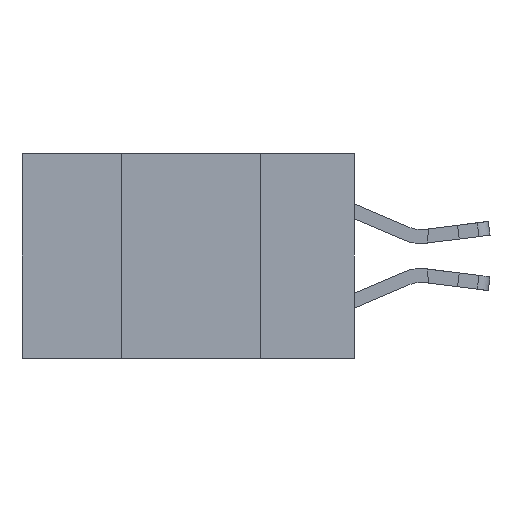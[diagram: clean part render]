
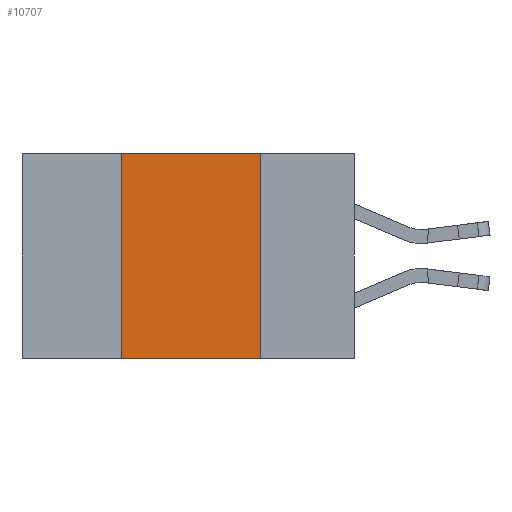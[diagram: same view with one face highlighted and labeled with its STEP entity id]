
A CAD part, left-side view. The second image highlights one B-rep face of the part: STEP entity #10707.
In plain terms, the highlighted planar face has unit normal (-1, 0, 0).
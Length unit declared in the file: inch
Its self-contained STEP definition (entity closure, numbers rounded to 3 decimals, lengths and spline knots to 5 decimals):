
#475 = VERTEX_POINT ( 'NONE', #1895 ) ;
#524 = CARTESIAN_POINT ( 'NONE',  ( 0., 0.42, -0.37 ) ) ;
#1473 = ORIENTED_EDGE ( 'NONE', *, *, #10453, .F. ) ;
#1657 = CARTESIAN_POINT ( 'NONE',  ( 0., 0.6, 0. ) ) ;
#1805 = FACE_OUTER_BOUND ( 'NONE', #2072, .T. ) ;
#1867 = ORIENTED_EDGE ( 'NONE', *, *, #7576, .F. ) ;
#1895 = CARTESIAN_POINT ( 'NONE',  ( 0., 0.17, 0. ) ) ;
#2072 = EDGE_LOOP ( 'NONE', ( #7737, #1867, #1473, #7550 ) ) ;
#2211 = LINE ( 'NONE', #5870, #7293 ) ;
#2310 = AXIS2_PLACEMENT_3D ( 'NONE', #5741, #8170, #5458 ) ;
#2349 = VECTOR ( 'NONE', #7899, 39.37008 ) ;
#3535 = EDGE_CURVE ( 'NONE', #8567, #10060, #2211, .T. ) ;
#3769 = EDGE_CURVE ( 'NONE', #475, #10060, #10664, .T. ) ;
#3781 = CARTESIAN_POINT ( 'NONE',  ( 0., 0.42, 0. ) ) ;
#3911 = PLANE ( 'NONE',  #2310 ) ;
#5458 = DIRECTION ( 'NONE',  ( 0., 0., -1. ) ) ;
#5741 = CARTESIAN_POINT ( 'NONE',  ( 0., 0.6, 0. ) ) ;
#5870 = CARTESIAN_POINT ( 'NONE',  ( 0., 0.6, -0.37 ) ) ;
#7293 = VECTOR ( 'NONE', #10392, 39.37008 ) ;
#7471 = LINE ( 'NONE', #524, #9683 ) ;
#7550 = ORIENTED_EDGE ( 'NONE', *, *, #3535, .T. ) ;
#7576 = EDGE_CURVE ( 'NONE', #8061, #475, #8795, .T. ) ;
#7656 = CARTESIAN_POINT ( 'NONE',  ( 0., 0.42, -0.37 ) ) ;
#7737 = ORIENTED_EDGE ( 'NONE', *, *, #3769, .F. ) ;
#7899 = DIRECTION ( 'NONE',  ( 0., 0., -1. ) ) ;
#8061 = VERTEX_POINT ( 'NONE', #3781 ) ;
#8170 = DIRECTION ( 'NONE',  ( 1., 0., 0. ) ) ;
#8567 = VERTEX_POINT ( 'NONE', #7656 ) ;
#8714 = VECTOR ( 'NONE', #10607, 39.37008 ) ;
#8795 = LINE ( 'NONE', #1657, #8714 ) ;
#9683 = VECTOR ( 'NONE', #10651, 39.37008 ) ;
#10060 = VERTEX_POINT ( 'NONE', #11563 ) ;
#10392 = DIRECTION ( 'NONE',  ( 0., -1., 0. ) ) ;
#10453 = EDGE_CURVE ( 'NONE', #8567, #8061, #7471, .T. ) ;
#10607 = DIRECTION ( 'NONE',  ( 0., -1., 0. ) ) ;
#10651 = DIRECTION ( 'NONE',  ( 0., 0., 1. ) ) ;
#10664 = LINE ( 'NONE', #10724, #2349 ) ;
#10707 = ADVANCED_FACE ( 'NONE', ( #1805 ), #3911, .F. ) ;
#10724 = CARTESIAN_POINT ( 'NONE',  ( 0., 0.17, -0.37 ) ) ;
#11563 = CARTESIAN_POINT ( 'NONE',  ( 0., 0.17, -0.37 ) ) ;
